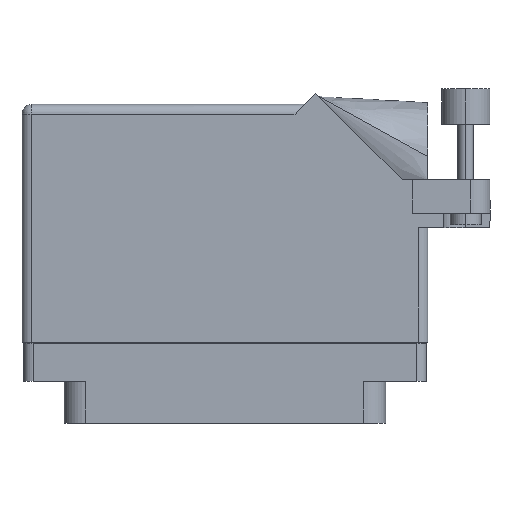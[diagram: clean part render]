
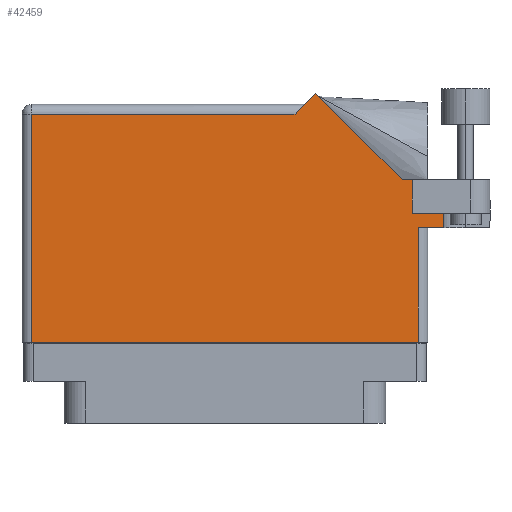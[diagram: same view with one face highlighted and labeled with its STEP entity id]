
A CAD part, front view. The second image highlights one B-rep face of the part: STEP entity #42459.
In plain terms, the highlighted face is planar.
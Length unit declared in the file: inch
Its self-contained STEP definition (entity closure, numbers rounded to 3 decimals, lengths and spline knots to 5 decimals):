
#432 = DIRECTION ( 'NONE',  ( 0., -1., 0. ) ) ;
#721 = ORIENTED_EDGE ( 'NONE', *, *, #29826, .T. ) ;
#2112 = CARTESIAN_POINT ( 'NONE',  ( 1.4075, 0.731, 0.455 ) ) ;
#2262 = FACE_OUTER_BOUND ( 'NONE', #22800, .T. ) ;
#3555 = EDGE_CURVE ( 'NONE', #38931, #45442, #39995, .T. ) ;
#4194 = CARTESIAN_POINT ( 'NONE',  ( 1.4075, 1.06177, 0.455 ) ) ;
#4426 = VERTEX_POINT ( 'NONE', #43805 ) ;
#4721 = ORIENTED_EDGE ( 'NONE', *, *, #3555, .T. ) ;
#4978 = ORIENTED_EDGE ( 'NONE', *, *, #10973, .F. ) ;
#5744 = VECTOR ( 'NONE', #21181, 39.37008 ) ;
#6513 = VECTOR ( 'NONE', #36978, 39.37008 ) ;
#7120 = LINE ( 'NONE', #10093, #45487 ) ;
#7534 = ORIENTED_EDGE ( 'NONE', *, *, #42595, .T. ) ;
#9763 = VECTOR ( 'NONE', #18908, 39.37008 ) ;
#9929 = DIRECTION ( 'NONE',  ( 0., 1., 0. ) ) ;
#10093 = CARTESIAN_POINT ( 'NONE',  ( 1.244, 0.637, 0.455 ) ) ;
#10154 = VERTEX_POINT ( 'NONE', #10392 ) ;
#10392 = CARTESIAN_POINT ( 'NONE',  ( -1.244, 1.368, 0.455 ) ) ;
#10973 = EDGE_CURVE ( 'NONE', #4426, #30006, #30932, .T. ) ;
#11329 = CARTESIAN_POINT ( 'NONE',  ( 1.244, 0.637, 0.455 ) ) ;
#13694 = VERTEX_POINT ( 'NONE', #30887 ) ;
#14929 = CARTESIAN_POINT ( 'NONE',  ( 0.513, 1.43, 0.455 ) ) ;
#15417 = ORIENTED_EDGE ( 'NONE', *, *, #47826, .T. ) ;
#15579 = VECTOR ( 'NONE', #432, 39.37008 ) ;
#15693 = CARTESIAN_POINT ( 'NONE',  ( 0.451, 1.368, 0.455 ) ) ;
#17104 = DIRECTION ( 'NONE',  ( 0., 0., -1. ) ) ;
#17620 = CARTESIAN_POINT ( 'NONE',  ( 1.206, 0.731, 0.455 ) ) ;
#17674 = VECTOR ( 'NONE', #19292, 39.37008 ) ;
#17917 = CARTESIAN_POINT ( 'NONE',  ( 1.14042, 0.944, 0.455 ) ) ;
#18169 = VECTOR ( 'NONE', #36278, 39.37008 ) ;
#18908 = DIRECTION ( 'NONE',  ( -1., 0., 0. ) ) ;
#19038 = LINE ( 'NONE', #45268, #41091 ) ;
#19220 = CARTESIAN_POINT ( 'NONE',  ( 1.706, 0.944, 0.455 ) ) ;
#19292 = DIRECTION ( 'NONE',  ( -0.707, 0.707, 0. ) ) ;
#21098 = ORIENTED_EDGE ( 'NONE', *, *, #23566, .T. ) ;
#21164 = DIRECTION ( 'NONE',  ( 1., 0., 0. ) ) ;
#21181 = DIRECTION ( 'NONE',  ( 0., -1., 0. ) ) ;
#21310 = ORIENTED_EDGE ( 'NONE', *, *, #39685, .T. ) ;
#22312 = CARTESIAN_POINT ( 'NONE',  ( -1.306, -0.1, 0.455 ) ) ;
#22671 = VECTOR ( 'NONE', #21164, 39.37008 ) ;
#22800 = EDGE_LOOP ( 'NONE', ( #4721, #31614, #7534, #31641, #4978, #25884, #42671, #21310, #721, #15417, #21098 ) ) ;
#23025 = DIRECTION ( 'NONE',  ( 0., 1., 0. ) ) ;
#23566 = EDGE_CURVE ( 'NONE', #10154, #38931, #45823, .T. ) ;
#24393 = CARTESIAN_POINT ( 'NONE',  ( -1.306, 1.43, 0.455 ) ) ;
#25722 = EDGE_CURVE ( 'NONE', #37097, #26971, #44065, .T. ) ;
#25884 = ORIENTED_EDGE ( 'NONE', *, *, #44241, .T. ) ;
#26546 = CARTESIAN_POINT ( 'NONE',  ( 1.244, -0.1, 0.455 ) ) ;
#26971 = VERTEX_POINT ( 'NONE', #17917 ) ;
#28168 = VERTEX_POINT ( 'NONE', #15693 ) ;
#29523 = VECTOR ( 'NONE', #36584, 39.37008 ) ;
#29826 = EDGE_CURVE ( 'NONE', #44554, #28168, #37890, .T. ) ;
#30006 = VERTEX_POINT ( 'NONE', #2112 ) ;
#30561 = CARTESIAN_POINT ( 'NONE',  ( 0.58371, 1.50071, 0.455 ) ) ;
#30887 = CARTESIAN_POINT ( 'NONE',  ( 1.4075, 0.637, 0.455 ) ) ;
#30932 = LINE ( 'NONE', #17620, #18169 ) ;
#31614 = ORIENTED_EDGE ( 'NONE', *, *, #36942, .T. ) ;
#31641 = ORIENTED_EDGE ( 'NONE', *, *, #43835, .F. ) ;
#31713 = PLANE ( 'NONE',  #41025 ) ;
#31919 = CARTESIAN_POINT ( 'NONE',  ( -1.244, -0.1, 0.455 ) ) ;
#32513 = CARTESIAN_POINT ( 'NONE',  ( -1.306, 1.368, 0.455 ) ) ;
#36278 = DIRECTION ( 'NONE',  ( 1., 0., 0. ) ) ;
#36584 = DIRECTION ( 'NONE',  ( 1., 0., 0. ) ) ;
#36942 = EDGE_CURVE ( 'NONE', #45442, #40009, #7120, .T. ) ;
#36978 = DIRECTION ( 'NONE',  ( -0.707, -0.707, 0. ) ) ;
#37097 = VERTEX_POINT ( 'NONE', #48100 ) ;
#37890 = LINE ( 'NONE', #14929, #6513 ) ;
#38931 = VERTEX_POINT ( 'NONE', #31919 ) ;
#39685 = EDGE_CURVE ( 'NONE', #26971, #44554, #44961, .T. ) ;
#39837 = CARTESIAN_POINT ( 'NONE',  ( -1.244, -0.1, 0.455 ) ) ;
#39995 = LINE ( 'NONE', #22312, #29523 ) ;
#40009 = VERTEX_POINT ( 'NONE', #11329 ) ;
#40130 = CARTESIAN_POINT ( 'NONE',  ( 1.306, 0.637, 0.455 ) ) ;
#40306 = VECTOR ( 'NONE', #47300, 39.37008 ) ;
#41025 = AXIS2_PLACEMENT_3D ( 'NONE', #24393, #17104, #43074 ) ;
#41091 = VECTOR ( 'NONE', #23025, 39.37008 ) ;
#42459 = ADVANCED_FACE ( 'NONE', ( #2262 ), #31713, .F. ) ;
#42595 = EDGE_CURVE ( 'NONE', #40009, #13694, #46475, .T. ) ;
#42618 = LINE ( 'NONE', #32513, #40306 ) ;
#42671 = ORIENTED_EDGE ( 'NONE', *, *, #25722, .T. ) ;
#42859 = LINE ( 'NONE', #4194, #15579 ) ;
#43074 = DIRECTION ( 'NONE',  ( -1., 0., 0. ) ) ;
#43805 = CARTESIAN_POINT ( 'NONE',  ( 1.206, 0.731, 0.455 ) ) ;
#43835 = EDGE_CURVE ( 'NONE', #30006, #13694, #42859, .T. ) ;
#44065 = LINE ( 'NONE', #19220, #9763 ) ;
#44241 = EDGE_CURVE ( 'NONE', #4426, #37097, #19038, .T. ) ;
#44554 = VERTEX_POINT ( 'NONE', #30561 ) ;
#44961 = LINE ( 'NONE', #45572, #17674 ) ;
#45268 = CARTESIAN_POINT ( 'NONE',  ( 1.206, 0.731, 0.455 ) ) ;
#45442 = VERTEX_POINT ( 'NONE', #26546 ) ;
#45487 = VECTOR ( 'NONE', #9929, 39.37008 ) ;
#45572 = CARTESIAN_POINT ( 'NONE',  ( 1.14042, 0.944, 0.455 ) ) ;
#45823 = LINE ( 'NONE', #39837, #5744 ) ;
#46475 = LINE ( 'NONE', #40130, #22671 ) ;
#47300 = DIRECTION ( 'NONE',  ( -1., 0., 0. ) ) ;
#47826 = EDGE_CURVE ( 'NONE', #28168, #10154, #42618, .T. ) ;
#48100 = CARTESIAN_POINT ( 'NONE',  ( 1.206, 0.944, 0.455 ) ) ;
